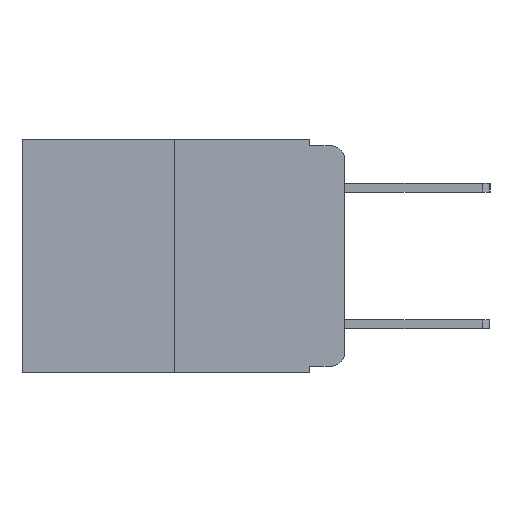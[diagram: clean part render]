
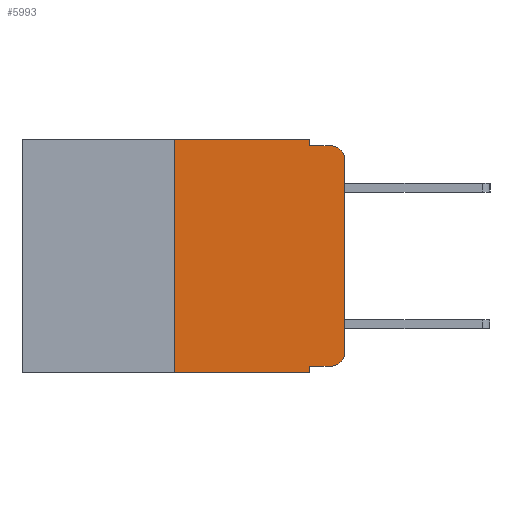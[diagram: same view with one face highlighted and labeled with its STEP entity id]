
A CAD part, left-side view. The second image highlights one B-rep face of the part: STEP entity #5993.
In plain terms, the highlighted planar face has unit normal (-1, 0, 0).
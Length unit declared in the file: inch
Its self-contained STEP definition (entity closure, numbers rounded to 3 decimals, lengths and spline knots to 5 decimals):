
#46 = ORIENTED_EDGE ( 'NONE', *, *, #10624, .T. ) ;
#411 = LINE ( 'NONE', #10518, #3946 ) ;
#891 = EDGE_CURVE ( 'NONE', #16752, #1137, #16845, .T. ) ;
#1137 = VERTEX_POINT ( 'NONE', #5430 ) ;
#1422 = CARTESIAN_POINT ( 'NONE',  ( 0., 0.051, 0. ) ) ;
#1506 = VERTEX_POINT ( 'NONE', #13052 ) ;
#2019 = VERTEX_POINT ( 'NONE', #7005 ) ;
#2423 = EDGE_CURVE ( 'NONE', #2019, #2448, #13874, .T. ) ;
#2448 = VERTEX_POINT ( 'NONE', #1422 ) ;
#2873 = EDGE_CURVE ( 'NONE', #1506, #16752, #6228, .T. ) ;
#3238 = ORIENTED_EDGE ( 'NONE', *, *, #4907, .F. ) ;
#3260 = VERTEX_POINT ( 'NONE', #4660 ) ;
#3427 = CARTESIAN_POINT ( 'NONE',  ( 0., 0.051, -0.01 ) ) ;
#3946 = VECTOR ( 'NONE', #7801, 39.37008 ) ;
#3960 = CARTESIAN_POINT ( 'NONE',  ( 0., 0., -0.03 ) ) ;
#4002 = VECTOR ( 'NONE', #4157, 39.37008 ) ;
#4107 = VECTOR ( 'NONE', #8803, 39.37008 ) ;
#4157 = DIRECTION ( 'NONE',  ( 0., 0., -1. ) ) ;
#4240 = CARTESIAN_POINT ( 'NONE',  ( 0., 0., 0. ) ) ;
#4660 = CARTESIAN_POINT ( 'NONE',  ( 0., 0.051, -0.343 ) ) ;
#4862 = VERTEX_POINT ( 'NONE', #3960 ) ;
#4907 = EDGE_CURVE ( 'NONE', #1506, #3260, #11800, .T. ) ;
#5430 = CARTESIAN_POINT ( 'NONE',  ( 0., 0., -0.313 ) ) ;
#5656 = CARTESIAN_POINT ( 'NONE',  ( 0., 0.02, -0.03 ) ) ;
#5766 = VECTOR ( 'NONE', #5884, 39.37008 ) ;
#5884 = DIRECTION ( 'NONE',  ( 0., -1., 0. ) ) ;
#5993 = ADVANCED_FACE ( 'NONE', ( #7903 ), #14279, .F. ) ;
#5997 = EDGE_LOOP ( 'NONE', ( #16381, #46, #14843, #6172, #10058, #11019, #12847, #3238, #11581, #16133 ) ) ;
#6172 = ORIENTED_EDGE ( 'NONE', *, *, #7925, .F. ) ;
#6215 = CIRCLE ( 'NONE', #12844, 0.02 ) ;
#6228 = LINE ( 'NONE', #15287, #5766 ) ;
#6564 = LINE ( 'NONE', #12644, #16687 ) ;
#6722 = CARTESIAN_POINT ( 'NONE',  ( 0., 0.473, 0. ) ) ;
#6895 = EDGE_CURVE ( 'NONE', #6958, #2019, #16410, .T. ) ;
#6958 = VERTEX_POINT ( 'NONE', #12676 ) ;
#7005 = CARTESIAN_POINT ( 'NONE',  ( 0., 0.25, 0. ) ) ;
#7163 = DIRECTION ( 'NONE',  ( 0., 0., -1. ) ) ;
#7801 = DIRECTION ( 'NONE',  ( 0., -1., 0. ) ) ;
#7903 = FACE_OUTER_BOUND ( 'NONE', #5997, .T. ) ;
#7925 = EDGE_CURVE ( 'NONE', #2448, #9853, #6564, .T. ) ;
#8246 = DIRECTION ( 'NONE',  ( 1., 0., 0. ) ) ;
#8636 = CARTESIAN_POINT ( 'NONE',  ( 0., 0.02, -0.333 ) ) ;
#8803 = DIRECTION ( 'NONE',  ( 0., 0., 1. ) ) ;
#8828 = DIRECTION ( 'NONE',  ( 0., 0., -1. ) ) ;
#8843 = DIRECTION ( 'NONE',  ( -1., 0., 0. ) ) ;
#8864 = CARTESIAN_POINT ( 'NONE',  ( 0., 0.02, -0.313 ) ) ;
#9146 = CARTESIAN_POINT ( 'NONE',  ( 0., 0.02, -0.01 ) ) ;
#9767 = EDGE_CURVE ( 'NONE', #9853, #14978, #411, .T. ) ;
#9853 = VERTEX_POINT ( 'NONE', #3427 ) ;
#10058 = ORIENTED_EDGE ( 'NONE', *, *, #2423, .F. ) ;
#10344 = EDGE_CURVE ( 'NONE', #6958, #3260, #16280, .T. ) ;
#10518 = CARTESIAN_POINT ( 'NONE',  ( 0., 0.051, -0.01 ) ) ;
#10624 = EDGE_CURVE ( 'NONE', #4862, #14978, #6215, .T. ) ;
#11019 = ORIENTED_EDGE ( 'NONE', *, *, #6895, .F. ) ;
#11420 = EDGE_CURVE ( 'NONE', #1137, #4862, #15412, .T. ) ;
#11581 = ORIENTED_EDGE ( 'NONE', *, *, #2873, .T. ) ;
#11800 = LINE ( 'NONE', #14533, #4002 ) ;
#12203 = AXIS2_PLACEMENT_3D ( 'NONE', #6722, #8246, #16492 ) ;
#12393 = DIRECTION ( 'NONE',  ( 0., 0., 1. ) ) ;
#12564 = CARTESIAN_POINT ( 'NONE',  ( 0., 0.473, -0.343 ) ) ;
#12644 = CARTESIAN_POINT ( 'NONE',  ( 0., 0.051, 0. ) ) ;
#12676 = CARTESIAN_POINT ( 'NONE',  ( 0., 0.25, -0.343 ) ) ;
#12815 = DIRECTION ( 'NONE',  ( 0., -1., 0. ) ) ;
#12844 = AXIS2_PLACEMENT_3D ( 'NONE', #5656, #14610, #7163 ) ;
#12847 = ORIENTED_EDGE ( 'NONE', *, *, #10344, .T. ) ;
#13052 = CARTESIAN_POINT ( 'NONE',  ( 0., 0.051, -0.333 ) ) ;
#13191 = VECTOR ( 'NONE', #12815, 39.37008 ) ;
#13336 = VECTOR ( 'NONE', #13682, 39.37008 ) ;
#13489 = VECTOR ( 'NONE', #12393, 39.37008 ) ;
#13682 = DIRECTION ( 'NONE',  ( 0., -1., 0. ) ) ;
#13874 = LINE ( 'NONE', #15670, #13191 ) ;
#14279 = PLANE ( 'NONE',  #12203 ) ;
#14533 = CARTESIAN_POINT ( 'NONE',  ( 0., 0.051, 0. ) ) ;
#14610 = DIRECTION ( 'NONE',  ( -1., 0., 0. ) ) ;
#14843 = ORIENTED_EDGE ( 'NONE', *, *, #9767, .F. ) ;
#14978 = VERTEX_POINT ( 'NONE', #9146 ) ;
#15287 = CARTESIAN_POINT ( 'NONE',  ( 0., 0.051, -0.333 ) ) ;
#15412 = LINE ( 'NONE', #4240, #13489 ) ;
#15670 = CARTESIAN_POINT ( 'NONE',  ( 0., 0.473, 0. ) ) ;
#15842 = CARTESIAN_POINT ( 'NONE',  ( 0., 0.25, 0. ) ) ;
#15995 = DIRECTION ( 'NONE',  ( 0., 0., -1. ) ) ;
#16133 = ORIENTED_EDGE ( 'NONE', *, *, #891, .T. ) ;
#16280 = LINE ( 'NONE', #12564, #13336 ) ;
#16381 = ORIENTED_EDGE ( 'NONE', *, *, #11420, .T. ) ;
#16410 = LINE ( 'NONE', #15842, #4107 ) ;
#16492 = DIRECTION ( 'NONE',  ( 0., 0., -1. ) ) ;
#16520 = AXIS2_PLACEMENT_3D ( 'NONE', #8864, #8843, #8828 ) ;
#16687 = VECTOR ( 'NONE', #15995, 39.37008 ) ;
#16752 = VERTEX_POINT ( 'NONE', #8636 ) ;
#16845 = CIRCLE ( 'NONE', #16520, 0.02 ) ;
